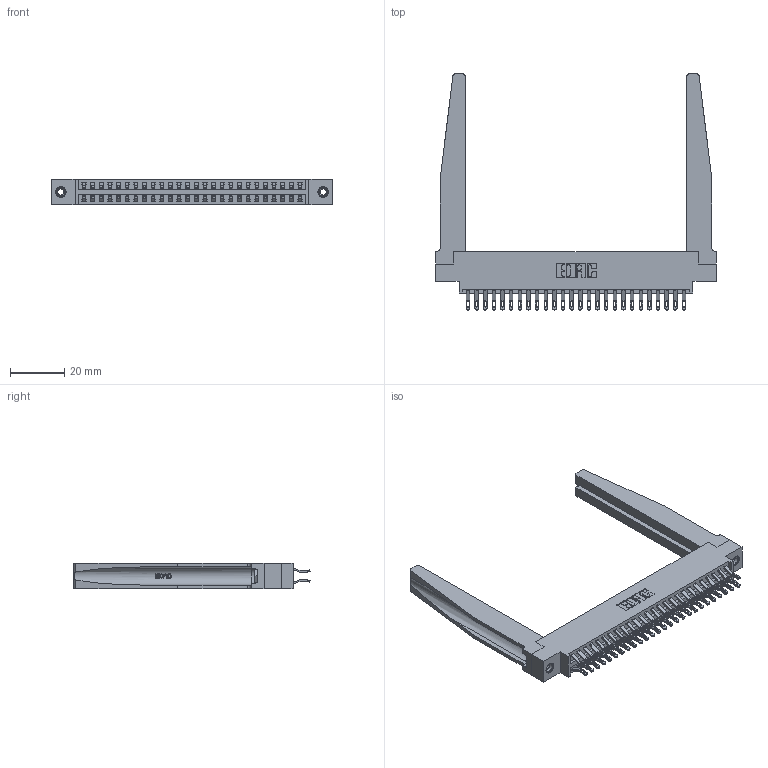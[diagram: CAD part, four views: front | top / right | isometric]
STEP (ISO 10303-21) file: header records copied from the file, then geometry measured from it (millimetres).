
FILE_DESCRIPTION (( 'STEP AP203' ), '1' );
FILE_NAME ('346-052-555-878.STEP', '2022-05-21T01:43:12', ( '' ), ( '' ), 'SwSTEP 2.0', 'SolidWorks 2020', '' );
FILE_SCHEMA (( 'CONFIG_CONTROL_DESIGN' ));
Length unit declared in the file: inch
Products named in the file (5): 345-292-001_555 Tail; 345-250-001_345-250-001-102; 346-052-555-878; 346 Part_0.170 Offset - 0.156 Dia-TH; 346-220-078_345-220-078
Assembly tree (57 placements, depth 2):
  346-052-555-878
    346 Part_0.170 Offset - 0.156 Dia-TH
    345-292-001_555 Tail  x52
    346-220-078_345-220-078  x2
    345-250-001_345-250-001-102  x2
Bounding box: 103.12 x 86.74 x 9.4 mm (x, y, z)
Volume: 16818.6 mm3; surface area: 20659.4 mm2
Topology: 57 solids, 57 shells, 3390 faces, 10501 edges, 6990 vertices
Faces by surface type: plane 1952, cylinder 1386, bspline 36, cone 12, torus 4
Entity records: 24744 total; most frequent: CARTESIAN_POINT 5079, ORIENTED_EDGE 3870, DIRECTION 3481, EDGE_CURVE 1935, VECTOR 1585, LINE 1585, VERTEX_POINT 1284, AXIS2_PLACEMENT_3D 948
